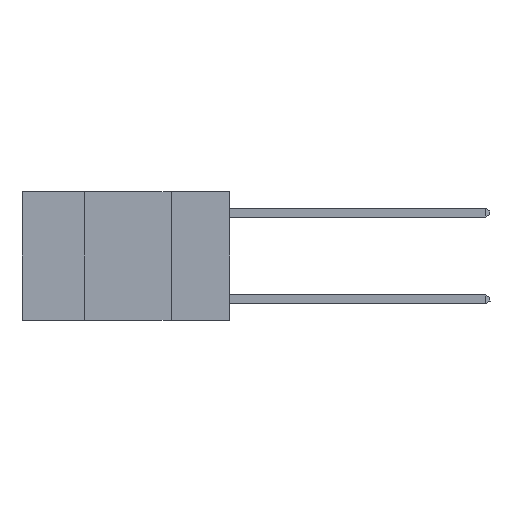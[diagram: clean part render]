
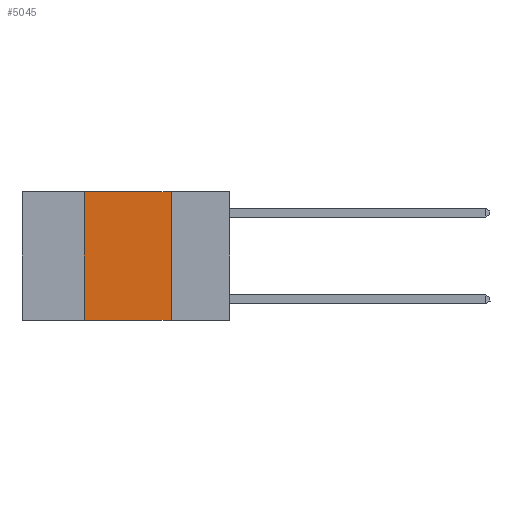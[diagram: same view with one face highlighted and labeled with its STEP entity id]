
A CAD part, left-side view. The second image highlights one B-rep face of the part: STEP entity #5045.
In plain terms, the highlighted planar face has unit normal (-1, 0, 0).
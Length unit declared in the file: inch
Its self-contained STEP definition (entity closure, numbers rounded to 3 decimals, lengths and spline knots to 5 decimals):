
#85 = VERTEX_POINT ( 'NONE', #8001 ) ;
#959 = VECTOR ( 'NONE', #11306, 39.37008 ) ;
#1159 = VERTEX_POINT ( 'NONE', #5122 ) ;
#1844 = FACE_OUTER_BOUND ( 'NONE', #17517, .T. ) ;
#2237 = LINE ( 'NONE', #3820, #16400 ) ;
#2272 = AXIS2_PLACEMENT_3D ( 'NONE', #7074, #16521, #8427 ) ;
#2524 = LINE ( 'NONE', #14369, #4545 ) ;
#2784 = CARTESIAN_POINT ( 'NONE',  ( 0., 0.42, -0.37 ) ) ;
#3083 = ORIENTED_EDGE ( 'NONE', *, *, #13814, .F. ) ;
#3401 = LINE ( 'NONE', #7765, #15215 ) ;
#3820 = CARTESIAN_POINT ( 'NONE',  ( 0., 0.17, 0. ) ) ;
#4048 = ORIENTED_EDGE ( 'NONE', *, *, #12921, .F. ) ;
#4051 = ORIENTED_EDGE ( 'NONE', *, *, #12023, .T. ) ;
#4545 = VECTOR ( 'NONE', #6202, 39.37008 ) ;
#4735 = LINE ( 'NONE', #9955, #959 ) ;
#5045 = ADVANCED_FACE ( 'NONE', ( #1844 ), #11140, .F. ) ;
#5107 = EDGE_CURVE ( 'NONE', #14824, #85, #4735, .T. ) ;
#5122 = CARTESIAN_POINT ( 'NONE',  ( 0., 0.17, -0.37 ) ) ;
#6202 = DIRECTION ( 'NONE',  ( 0., -1., 0. ) ) ;
#7074 = CARTESIAN_POINT ( 'NONE',  ( 0., 0.6, 0. ) ) ;
#7765 = CARTESIAN_POINT ( 'NONE',  ( 0., 0.42, 0. ) ) ;
#8001 = CARTESIAN_POINT ( 'NONE',  ( 0., 0.17, 0. ) ) ;
#8024 = DIRECTION ( 'NONE',  ( 0., 0., -1. ) ) ;
#8427 = DIRECTION ( 'NONE',  ( 0., 0., -1. ) ) ;
#9955 = CARTESIAN_POINT ( 'NONE',  ( 0., 0.6, 0. ) ) ;
#11140 = PLANE ( 'NONE',  #2272 ) ;
#11306 = DIRECTION ( 'NONE',  ( 0., -1., 0. ) ) ;
#12023 = EDGE_CURVE ( 'NONE', #14625, #1159, #2524, .T. ) ;
#12921 = EDGE_CURVE ( 'NONE', #14625, #14824, #3401, .T. ) ;
#13217 = ORIENTED_EDGE ( 'NONE', *, *, #5107, .F. ) ;
#13814 = EDGE_CURVE ( 'NONE', #85, #1159, #2237, .T. ) ;
#14369 = CARTESIAN_POINT ( 'NONE',  ( 0., 0.6, -0.37 ) ) ;
#14625 = VERTEX_POINT ( 'NONE', #2784 ) ;
#14824 = VERTEX_POINT ( 'NONE', #16760 ) ;
#15215 = VECTOR ( 'NONE', #17151, 39.37008 ) ;
#16400 = VECTOR ( 'NONE', #8024, 39.37008 ) ;
#16521 = DIRECTION ( 'NONE',  ( 1., 0., 0. ) ) ;
#16760 = CARTESIAN_POINT ( 'NONE',  ( 0., 0.42, 0. ) ) ;
#17151 = DIRECTION ( 'NONE',  ( 0., 0., 1. ) ) ;
#17517 = EDGE_LOOP ( 'NONE', ( #3083, #13217, #4048, #4051 ) ) ;
